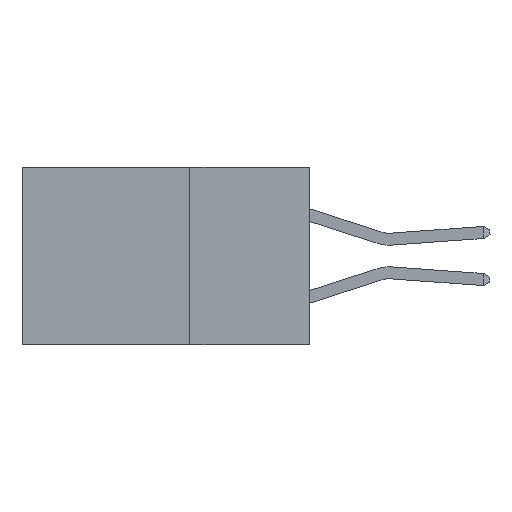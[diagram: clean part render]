
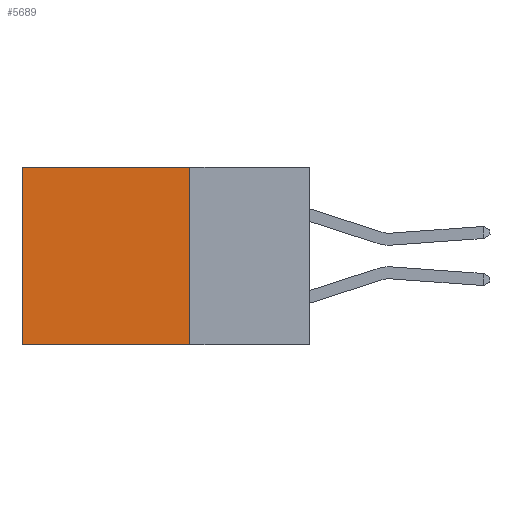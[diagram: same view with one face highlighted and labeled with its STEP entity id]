
A CAD part, left-side view. The second image highlights one B-rep face of the part: STEP entity #5689.
In plain terms, the highlighted planar face has unit normal (-1, 0, 0).
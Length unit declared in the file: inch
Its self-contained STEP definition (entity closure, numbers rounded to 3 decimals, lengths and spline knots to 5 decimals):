
#1260 = AXIS2_PLACEMENT_3D ( 'NONE', #6329, #5930, #3269 ) ;
#1528 = DIRECTION ( 'NONE',  ( 0., 1., 0. ) ) ;
#2589 = VERTEX_POINT ( 'NONE', #11323 ) ;
#3088 = ORIENTED_EDGE ( 'NONE', *, *, #14006, .T. ) ;
#3269 = DIRECTION ( 'NONE',  ( 0., 0., -1. ) ) ;
#3679 = LINE ( 'NONE', #7557, #12388 ) ;
#3821 = DIRECTION ( 'NONE',  ( 0., 0., -1. ) ) ;
#3868 = CARTESIAN_POINT ( 'NONE',  ( 0.298, 0.25, 0. ) ) ;
#4331 = EDGE_CURVE ( 'NONE', #2589, #13122, #10461, .T. ) ;
#4476 = CARTESIAN_POINT ( 'NONE',  ( 0.298, 0.25, -0.37 ) ) ;
#4814 = CARTESIAN_POINT ( 'NONE',  ( 0.298, 0.25, 0. ) ) ;
#5372 = CARTESIAN_POINT ( 'NONE',  ( 0.298, 0.6, 0. ) ) ;
#5689 = ADVANCED_FACE ( 'NONE', ( #11674 ), #6430, .F. ) ;
#5930 = DIRECTION ( 'NONE',  ( 1., 0., 0. ) ) ;
#6075 = ORIENTED_EDGE ( 'NONE', *, *, #8539, .F. ) ;
#6090 = LINE ( 'NONE', #14151, #8757 ) ;
#6329 = CARTESIAN_POINT ( 'NONE',  ( 0.298, 0.25, 0. ) ) ;
#6430 = PLANE ( 'NONE',  #1260 ) ;
#6463 = EDGE_LOOP ( 'NONE', ( #3088, #6075, #9101, #6787 ) ) ;
#6787 = ORIENTED_EDGE ( 'NONE', *, *, #11830, .T. ) ;
#6952 = VERTEX_POINT ( 'NONE', #5372 ) ;
#7088 = VECTOR ( 'NONE', #3821, 39.37008 ) ;
#7557 = CARTESIAN_POINT ( 'NONE',  ( 0.298, 0.6, 0. ) ) ;
#7840 = LINE ( 'NONE', #4814, #10126 ) ;
#8500 = DIRECTION ( 'NONE',  ( 0., 1., 0. ) ) ;
#8539 = EDGE_CURVE ( 'NONE', #13122, #10672, #6090, .T. ) ;
#8599 = DIRECTION ( 'NONE',  ( 0., 0., -1. ) ) ;
#8757 = VECTOR ( 'NONE', #8500, 39.37008 ) ;
#9101 = ORIENTED_EDGE ( 'NONE', *, *, #4331, .F. ) ;
#10126 = VECTOR ( 'NONE', #1528, 39.37008 ) ;
#10461 = LINE ( 'NONE', #3868, #7088 ) ;
#10672 = VERTEX_POINT ( 'NONE', #11469 ) ;
#11323 = CARTESIAN_POINT ( 'NONE',  ( 0.298, 0.25, 0. ) ) ;
#11469 = CARTESIAN_POINT ( 'NONE',  ( 0.298, 0.6, -0.37 ) ) ;
#11674 = FACE_OUTER_BOUND ( 'NONE', #6463, .T. ) ;
#11830 = EDGE_CURVE ( 'NONE', #2589, #6952, #7840, .T. ) ;
#12388 = VECTOR ( 'NONE', #8599, 39.37008 ) ;
#13122 = VERTEX_POINT ( 'NONE', #4476 ) ;
#14006 = EDGE_CURVE ( 'NONE', #6952, #10672, #3679, .T. ) ;
#14151 = CARTESIAN_POINT ( 'NONE',  ( 0.298, 0.25, -0.37 ) ) ;
